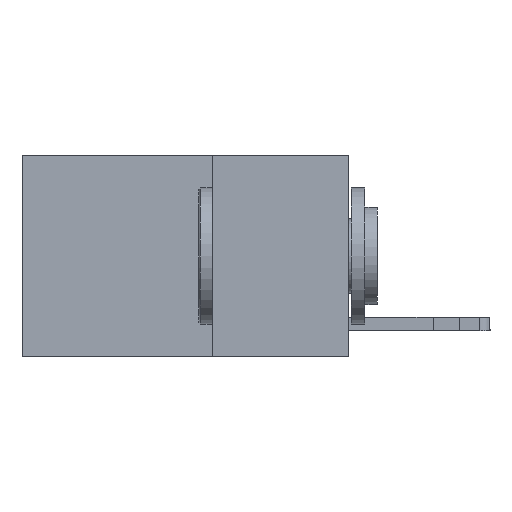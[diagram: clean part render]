
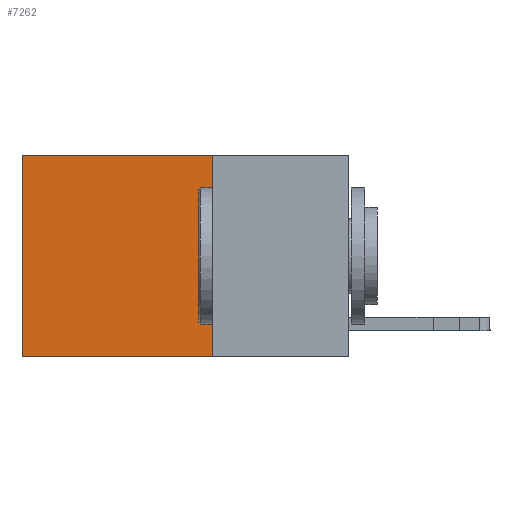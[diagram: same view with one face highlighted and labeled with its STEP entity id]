
A CAD part, left-side view. The second image highlights one B-rep face of the part: STEP entity #7262.
In plain terms, the highlighted planar face has unit normal (-1, 0, 0).
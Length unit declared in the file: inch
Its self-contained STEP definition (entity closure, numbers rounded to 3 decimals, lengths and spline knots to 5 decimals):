
#15 = FACE_OUTER_BOUND ( 'NONE', #14231, .T. ) ;
#137 = EDGE_CURVE ( 'NONE', #3929, #8249, #3494, .T. ) ;
#1095 = DIRECTION ( 'NONE',  ( 0., 0., -1. ) ) ;
#1190 = LINE ( 'NONE', #11789, #10310 ) ;
#1263 = CARTESIAN_POINT ( 'NONE',  ( 0.2625, 0.25, 0. ) ) ;
#1675 = AXIS2_PLACEMENT_3D ( 'NONE', #1263, #10696, #1095 ) ;
#3167 = EDGE_CURVE ( 'NONE', #8249, #9287, #15143, .T. ) ;
#3171 = CARTESIAN_POINT ( 'NONE',  ( 0.2625, 0.6, -0.37 ) ) ;
#3273 = DIRECTION ( 'NONE',  ( 0., 0., -1. ) ) ;
#3391 = CARTESIAN_POINT ( 'NONE',  ( 0.2625, 0.6, 0. ) ) ;
#3491 = LINE ( 'NONE', #9507, #4826 ) ;
#3494 = LINE ( 'NONE', #9435, #13968 ) ;
#3929 = VERTEX_POINT ( 'NONE', #10287 ) ;
#4394 = VECTOR ( 'NONE', #9048, 39.37008 ) ;
#4826 = VECTOR ( 'NONE', #14422, 39.37008 ) ;
#6093 = PLANE ( 'NONE',  #1675 ) ;
#6097 = ORIENTED_EDGE ( 'NONE', *, *, #3167, .T. ) ;
#7262 = ADVANCED_FACE ( 'NONE', ( #15 ), #6093, .F. ) ;
#8249 = VERTEX_POINT ( 'NONE', #3391 ) ;
#9048 = DIRECTION ( 'NONE',  ( 0., 0., -1. ) ) ;
#9071 = EDGE_CURVE ( 'NONE', #14102, #9287, #3491, .T. ) ;
#9279 = CARTESIAN_POINT ( 'NONE',  ( 0.2625, 0.6, 0. ) ) ;
#9287 = VERTEX_POINT ( 'NONE', #3171 ) ;
#9435 = CARTESIAN_POINT ( 'NONE',  ( 0.2625, 0.25, 0. ) ) ;
#9503 = ORIENTED_EDGE ( 'NONE', *, *, #137, .T. ) ;
#9507 = CARTESIAN_POINT ( 'NONE',  ( 0.2625, 0.25, -0.37 ) ) ;
#10119 = ORIENTED_EDGE ( 'NONE', *, *, #9071, .F. ) ;
#10287 = CARTESIAN_POINT ( 'NONE',  ( 0.2625, 0.25, 0. ) ) ;
#10310 = VECTOR ( 'NONE', #3273, 39.37008 ) ;
#10501 = EDGE_CURVE ( 'NONE', #3929, #14102, #1190, .T. ) ;
#10696 = DIRECTION ( 'NONE',  ( 1., 0., 0. ) ) ;
#11773 = DIRECTION ( 'NONE',  ( 0., 1., 0. ) ) ;
#11789 = CARTESIAN_POINT ( 'NONE',  ( 0.2625, 0.25, 0. ) ) ;
#12364 = ORIENTED_EDGE ( 'NONE', *, *, #10501, .F. ) ;
#13968 = VECTOR ( 'NONE', #11773, 39.37008 ) ;
#14102 = VERTEX_POINT ( 'NONE', #15139 ) ;
#14231 = EDGE_LOOP ( 'NONE', ( #6097, #10119, #12364, #9503 ) ) ;
#14422 = DIRECTION ( 'NONE',  ( 0., 1., 0. ) ) ;
#15139 = CARTESIAN_POINT ( 'NONE',  ( 0.2625, 0.25, -0.37 ) ) ;
#15143 = LINE ( 'NONE', #9279, #4394 ) ;
